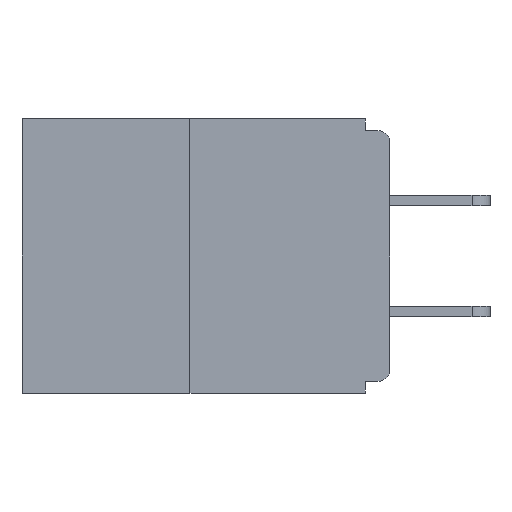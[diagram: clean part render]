
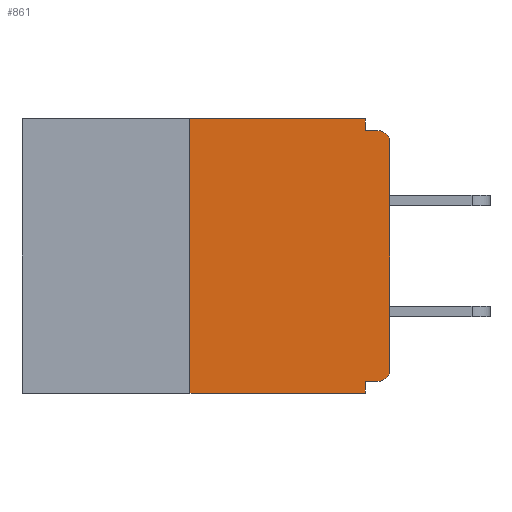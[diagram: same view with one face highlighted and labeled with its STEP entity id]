
A CAD part, left-side view. The second image highlights one B-rep face of the part: STEP entity #861.
In plain terms, the highlighted planar face has unit normal (-1, 0, 0).
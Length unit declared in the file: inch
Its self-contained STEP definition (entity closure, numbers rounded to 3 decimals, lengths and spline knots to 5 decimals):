
#351 = CIRCLE ( 'NONE', #4498, 0.015 ) ;
#374 = CARTESIAN_POINT ( 'NONE',  ( 0., 0.46, 0. ) ) ;
#438 = ORIENTED_EDGE ( 'NONE', *, *, #8540, .F. ) ;
#861 = ADVANCED_FACE ( 'NONE', ( #19096 ), #20079, .F. ) ;
#1008 = CARTESIAN_POINT ( 'NONE',  ( 0., 0.25, 0. ) ) ;
#1317 = CARTESIAN_POINT ( 'NONE',  ( 0., 0.25, -0.343 ) ) ;
#1327 = LINE ( 'NONE', #1008, #22672 ) ;
#1373 = DIRECTION ( 'NONE',  ( 0., 0., 1. ) ) ;
#2106 = VERTEX_POINT ( 'NONE', #13764 ) ;
#2472 = DIRECTION ( 'NONE',  ( 0., 0., -1. ) ) ;
#2850 = VERTEX_POINT ( 'NONE', #1317 ) ;
#3168 = LINE ( 'NONE', #15979, #21746 ) ;
#3545 = CARTESIAN_POINT ( 'NONE',  ( 0., 0.031, -0.328 ) ) ;
#3646 = EDGE_CURVE ( 'NONE', #20499, #16960, #8526, .T. ) ;
#4143 = VECTOR ( 'NONE', #16609, 39.37008 ) ;
#4498 = AXIS2_PLACEMENT_3D ( 'NONE', #19594, #16081, #17886 ) ;
#4805 = EDGE_CURVE ( 'NONE', #2850, #19574, #3168, .T. ) ;
#4957 = DIRECTION ( 'NONE',  ( 0., 0., -1. ) ) ;
#5601 = DIRECTION ( 'NONE',  ( 1., 0., 0. ) ) ;
#5851 = DIRECTION ( 'NONE',  ( 0., -1., 0. ) ) ;
#5979 = CARTESIAN_POINT ( 'NONE',  ( 0., 0.031, -0.343 ) ) ;
#7134 = EDGE_CURVE ( 'NONE', #17936, #19574, #17133, .T. ) ;
#7342 = DIRECTION ( 'NONE',  ( 0., -1., 0. ) ) ;
#8526 = CIRCLE ( 'NONE', #13740, 0.015 ) ;
#8540 = EDGE_CURVE ( 'NONE', #13738, #2106, #21584, .T. ) ;
#8774 = CARTESIAN_POINT ( 'NONE',  ( 0., 0.015, -0.328 ) ) ;
#8832 = CARTESIAN_POINT ( 'NONE',  ( 0., 0.015, -0.03 ) ) ;
#10594 = EDGE_LOOP ( 'NONE', ( #22972, #20676, #14126, #20592, #14252, #21620, #20735, #12965, #11795, #438 ) ) ;
#10832 = VECTOR ( 'NONE', #4957, 39.37008 ) ;
#11314 = EDGE_CURVE ( 'NONE', #14304, #23095, #351, .T. ) ;
#11795 = ORIENTED_EDGE ( 'NONE', *, *, #17055, .F. ) ;
#11848 = VECTOR ( 'NONE', #5851, 39.37008 ) ;
#11914 = VECTOR ( 'NONE', #1373, 39.37008 ) ;
#12939 = CARTESIAN_POINT ( 'NONE',  ( 0., 0.46, 0. ) ) ;
#12965 = ORIENTED_EDGE ( 'NONE', *, *, #3646, .T. ) ;
#13426 = EDGE_CURVE ( 'NONE', #14304, #17936, #22424, .T. ) ;
#13738 = VERTEX_POINT ( 'NONE', #23153 ) ;
#13740 = AXIS2_PLACEMENT_3D ( 'NONE', #8832, #14284, #23065 ) ;
#13764 = CARTESIAN_POINT ( 'NONE',  ( 0., 0.031, -0.015 ) ) ;
#13878 = LINE ( 'NONE', #22824, #11914 ) ;
#13915 = EDGE_CURVE ( 'NONE', #2850, #21980, #1327, .T. ) ;
#14125 = LINE ( 'NONE', #20186, #11848 ) ;
#14126 = ORIENTED_EDGE ( 'NONE', *, *, #4805, .T. ) ;
#14252 = ORIENTED_EDGE ( 'NONE', *, *, #13426, .F. ) ;
#14284 = DIRECTION ( 'NONE',  ( -1., 0., 0. ) ) ;
#14304 = VERTEX_POINT ( 'NONE', #8774 ) ;
#14666 = DIRECTION ( 'NONE',  ( 0., 0., -1. ) ) ;
#15467 = CARTESIAN_POINT ( 'NONE',  ( 0., 0., -0.03 ) ) ;
#15675 = CARTESIAN_POINT ( 'NONE',  ( 0., 0.031, 0. ) ) ;
#15979 = CARTESIAN_POINT ( 'NONE',  ( 0., 0.46, -0.343 ) ) ;
#16081 = DIRECTION ( 'NONE',  ( -1., 0., 0. ) ) ;
#16356 = VECTOR ( 'NONE', #7342, 39.37008 ) ;
#16609 = DIRECTION ( 'NONE',  ( 0., 1., 0. ) ) ;
#16649 = LINE ( 'NONE', #12939, #16356 ) ;
#16960 = VERTEX_POINT ( 'NONE', #18223 ) ;
#17055 = EDGE_CURVE ( 'NONE', #2106, #16960, #14125, .T. ) ;
#17133 = LINE ( 'NONE', #5979, #22193 ) ;
#17827 = CARTESIAN_POINT ( 'NONE',  ( 0., 0.25, 0. ) ) ;
#17886 = DIRECTION ( 'NONE',  ( 0., 0., -1. ) ) ;
#17936 = VERTEX_POINT ( 'NONE', #3545 ) ;
#18223 = CARTESIAN_POINT ( 'NONE',  ( 0., 0.015, -0.015 ) ) ;
#19096 = FACE_OUTER_BOUND ( 'NONE', #10594, .T. ) ;
#19181 = DIRECTION ( 'NONE',  ( 0., -1., 0. ) ) ;
#19574 = VERTEX_POINT ( 'NONE', #23243 ) ;
#19594 = CARTESIAN_POINT ( 'NONE',  ( 0., 0.015, -0.313 ) ) ;
#19883 = CARTESIAN_POINT ( 'NONE',  ( 0., 0., -0.328 ) ) ;
#20061 = AXIS2_PLACEMENT_3D ( 'NONE', #374, #5601, #14666 ) ;
#20079 = PLANE ( 'NONE',  #20061 ) ;
#20186 = CARTESIAN_POINT ( 'NONE',  ( 0., 0., -0.015 ) ) ;
#20337 = CARTESIAN_POINT ( 'NONE',  ( 0., 0., -0.313 ) ) ;
#20499 = VERTEX_POINT ( 'NONE', #15467 ) ;
#20515 = DIRECTION ( 'NONE',  ( 0., 0., 1. ) ) ;
#20569 = EDGE_CURVE ( 'NONE', #23095, #20499, #13878, .T. ) ;
#20592 = ORIENTED_EDGE ( 'NONE', *, *, #7134, .F. ) ;
#20676 = ORIENTED_EDGE ( 'NONE', *, *, #13915, .F. ) ;
#20735 = ORIENTED_EDGE ( 'NONE', *, *, #20569, .T. ) ;
#21584 = LINE ( 'NONE', #15675, #10832 ) ;
#21620 = ORIENTED_EDGE ( 'NONE', *, *, #11314, .T. ) ;
#21746 = VECTOR ( 'NONE', #19181, 39.37008 ) ;
#21980 = VERTEX_POINT ( 'NONE', #17827 ) ;
#22193 = VECTOR ( 'NONE', #2472, 39.37008 ) ;
#22395 = EDGE_CURVE ( 'NONE', #21980, #13738, #16649, .T. ) ;
#22424 = LINE ( 'NONE', #19883, #4143 ) ;
#22672 = VECTOR ( 'NONE', #20515, 39.37008 ) ;
#22824 = CARTESIAN_POINT ( 'NONE',  ( 0., 0., 0. ) ) ;
#22972 = ORIENTED_EDGE ( 'NONE', *, *, #22395, .F. ) ;
#23065 = DIRECTION ( 'NONE',  ( 0., 0., -1. ) ) ;
#23095 = VERTEX_POINT ( 'NONE', #20337 ) ;
#23153 = CARTESIAN_POINT ( 'NONE',  ( 0., 0.031, 0. ) ) ;
#23243 = CARTESIAN_POINT ( 'NONE',  ( 0., 0.031, -0.343 ) ) ;
